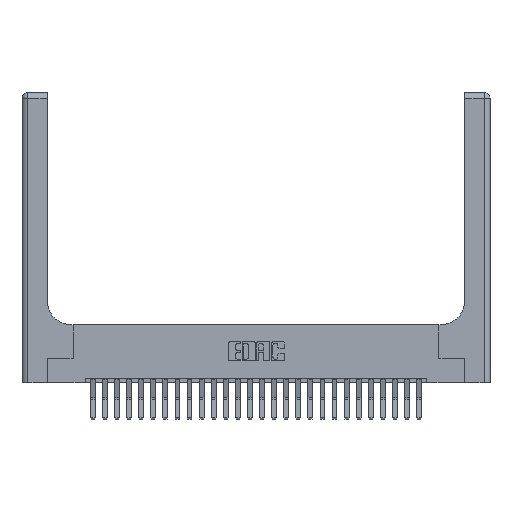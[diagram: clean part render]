
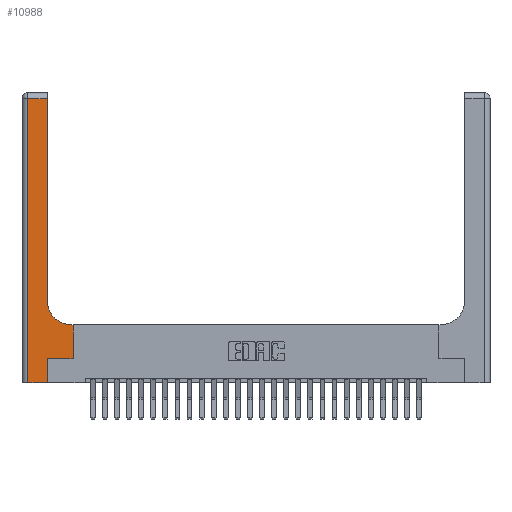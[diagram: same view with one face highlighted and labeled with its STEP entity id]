
A CAD part, top view. The second image highlights one B-rep face of the part: STEP entity #10988.
In plain terms, the highlighted planar face has unit normal (0, 0, 1).
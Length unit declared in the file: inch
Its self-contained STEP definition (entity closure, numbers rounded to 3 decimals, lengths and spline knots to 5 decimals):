
#24 = VERTEX_POINT ( 'NONE', #17411 ) ;
#90 = DIRECTION ( 'NONE',  ( 0., 0., -1. ) ) ;
#208 = DIRECTION ( 'NONE',  ( -1., 0., 0. ) ) ;
#254 = DIRECTION ( 'NONE',  ( 1., 0., 0. ) ) ;
#374 = LINE ( 'NONE', #3280, #24053 ) ;
#618 = EDGE_CURVE ( 'NONE', #25401, #9029, #8830, .T. ) ;
#659 = CIRCLE ( 'NONE', #17435, 0.25 ) ;
#2380 = VECTOR ( 'NONE', #208, 39.37008 ) ;
#2417 = CARTESIAN_POINT ( 'NONE',  ( 0.528, 0.25, 0.37 ) ) ;
#2641 = VERTEX_POINT ( 'NONE', #22864 ) ;
#2985 = ORIENTED_EDGE ( 'NONE', *, *, #17783, .T. ) ;
#3026 = EDGE_CURVE ( 'NONE', #2641, #24, #374, .T. ) ;
#3280 = CARTESIAN_POINT ( 'NONE',  ( 0.265, 0.25, 0.37 ) ) ;
#3300 = VERTEX_POINT ( 'NONE', #3415 ) ;
#3411 = EDGE_CURVE ( 'NONE', #3300, #18750, #12986, .T. ) ;
#3415 = CARTESIAN_POINT ( 'NONE',  ( 0.06, 0., 0.37 ) ) ;
#4004 = CARTESIAN_POINT ( 'NONE',  ( 0.26, 0.85, 0.37 ) ) ;
#4521 = DIRECTION ( 'NONE',  ( 0., -1., 0. ) ) ;
#4539 = ORIENTED_EDGE ( 'NONE', *, *, #618, .T. ) ;
#4574 = CARTESIAN_POINT ( 'NONE',  ( 0.26, 3., 0.37 ) ) ;
#5013 = ORIENTED_EDGE ( 'NONE', *, *, #24818, .T. ) ;
#5739 = EDGE_CURVE ( 'NONE', #9029, #10672, #659, .T. ) ;
#5987 = FACE_OUTER_BOUND ( 'NONE', #15971, .T. ) ;
#6126 = ORIENTED_EDGE ( 'NONE', *, *, #11807, .T. ) ;
#6318 = EDGE_CURVE ( 'NONE', #21696, #3300, #9859, .T. ) ;
#6343 = VECTOR ( 'NONE', #11876, 39.37008 ) ;
#6698 = CARTESIAN_POINT ( 'NONE',  ( 0.26, 2.94, 0.37 ) ) ;
#7881 = ORIENTED_EDGE ( 'NONE', *, *, #8032, .T. ) ;
#7994 = ORIENTED_EDGE ( 'NONE', *, *, #5739, .T. ) ;
#8032 = EDGE_CURVE ( 'NONE', #24, #25401, #23298, .T. ) ;
#8830 = LINE ( 'NONE', #23954, #11916 ) ;
#8967 = VECTOR ( 'NONE', #4521, 39.37008 ) ;
#9029 = VERTEX_POINT ( 'NONE', #24202 ) ;
#9214 = DIRECTION ( 'NONE',  ( -1., 0., 0. ) ) ;
#9859 = LINE ( 'NONE', #14293, #8967 ) ;
#9944 = DIRECTION ( 'NONE',  ( 1., 0., 0. ) ) ;
#10672 = VERTEX_POINT ( 'NONE', #4004 ) ;
#10988 = ADVANCED_FACE ( 'NONE', ( #5987 ), #17019, .F. ) ;
#11570 = AXIS2_PLACEMENT_3D ( 'NONE', #13334, #24837, #9214 ) ;
#11807 = EDGE_CURVE ( 'NONE', #10672, #13809, #14894, .T. ) ;
#11876 = DIRECTION ( 'NONE',  ( 0., 1., 0. ) ) ;
#11916 = VECTOR ( 'NONE', #12195, 39.37008 ) ;
#12195 = DIRECTION ( 'NONE',  ( -1., 0., 0. ) ) ;
#12986 = LINE ( 'NONE', #21830, #24953 ) ;
#13334 = CARTESIAN_POINT ( 'NONE',  ( 0., 3., 0.37 ) ) ;
#13809 = VERTEX_POINT ( 'NONE', #6698 ) ;
#14293 = CARTESIAN_POINT ( 'NONE',  ( 0.06, 3., 0.37 ) ) ;
#14650 = CARTESIAN_POINT ( 'NONE',  ( 0., 2.94, 0.37 ) ) ;
#14894 = LINE ( 'NONE', #4574, #6343 ) ;
#14918 = LINE ( 'NONE', #21519, #16158 ) ;
#15738 = CARTESIAN_POINT ( 'NONE',  ( 0.51, 0.85, 0.37 ) ) ;
#15739 = CARTESIAN_POINT ( 'NONE',  ( 0.528, 0.6, 0.37 ) ) ;
#15971 = EDGE_LOOP ( 'NONE', ( #6126, #2985, #25357, #16435, #5013, #17849, #7881, #4539, #7994 ) ) ;
#16104 = CARTESIAN_POINT ( 'NONE',  ( 0.06, 2.94, 0.37 ) ) ;
#16158 = VECTOR ( 'NONE', #23585, 39.37008 ) ;
#16435 = ORIENTED_EDGE ( 'NONE', *, *, #3411, .T. ) ;
#17019 = PLANE ( 'NONE',  #11570 ) ;
#17411 = CARTESIAN_POINT ( 'NONE',  ( 0.528, 0.25, 0.37 ) ) ;
#17435 = AXIS2_PLACEMENT_3D ( 'NONE', #15738, #90, #254 ) ;
#17525 = CARTESIAN_POINT ( 'NONE',  ( 0.265, 0., 0.37 ) ) ;
#17783 = EDGE_CURVE ( 'NONE', #13809, #21696, #19263, .T. ) ;
#17849 = ORIENTED_EDGE ( 'NONE', *, *, #3026, .T. ) ;
#18750 = VERTEX_POINT ( 'NONE', #17525 ) ;
#19263 = LINE ( 'NONE', #14650, #2380 ) ;
#19783 = DIRECTION ( 'NONE',  ( 1., 0., 0. ) ) ;
#20748 = DIRECTION ( 'NONE',  ( 0., 1., 0. ) ) ;
#21519 = CARTESIAN_POINT ( 'NONE',  ( 0.265, 0., 0.37 ) ) ;
#21696 = VERTEX_POINT ( 'NONE', #16104 ) ;
#21830 = CARTESIAN_POINT ( 'NONE',  ( 0., 0., 0.37 ) ) ;
#22673 = VECTOR ( 'NONE', #20748, 39.37008 ) ;
#22864 = CARTESIAN_POINT ( 'NONE',  ( 0.265, 0.25, 0.37 ) ) ;
#23298 = LINE ( 'NONE', #2417, #22673 ) ;
#23585 = DIRECTION ( 'NONE',  ( 0., 1., 0. ) ) ;
#23954 = CARTESIAN_POINT ( 'NONE',  ( 0.26, 0.6, 0.37 ) ) ;
#24053 = VECTOR ( 'NONE', #9944, 39.37008 ) ;
#24202 = CARTESIAN_POINT ( 'NONE',  ( 0.51, 0.6, 0.37 ) ) ;
#24818 = EDGE_CURVE ( 'NONE', #18750, #2641, #14918, .T. ) ;
#24837 = DIRECTION ( 'NONE',  ( 0., 0., -1. ) ) ;
#24953 = VECTOR ( 'NONE', #19783, 39.37008 ) ;
#25357 = ORIENTED_EDGE ( 'NONE', *, *, #6318, .T. ) ;
#25401 = VERTEX_POINT ( 'NONE', #15739 ) ;
